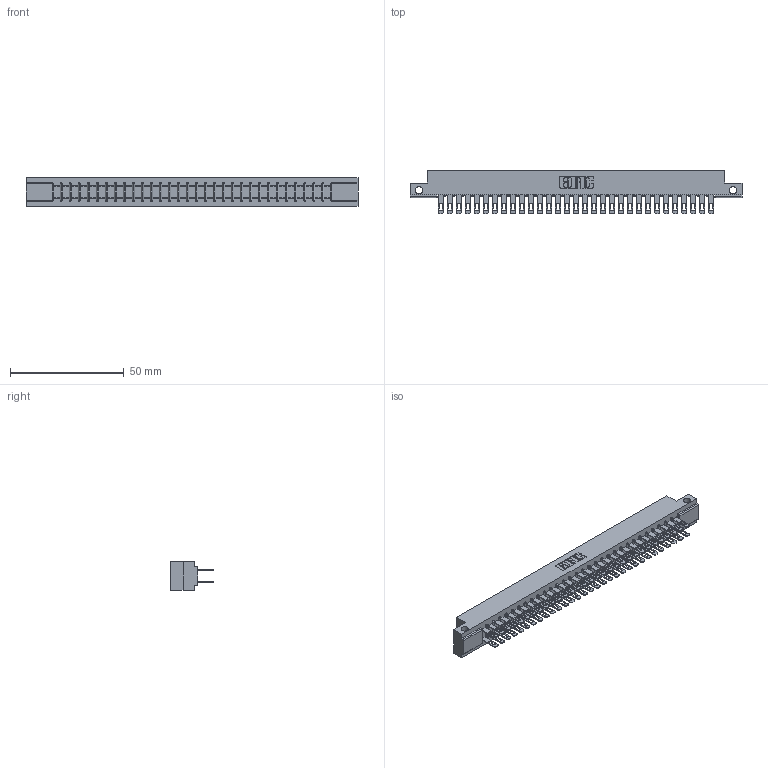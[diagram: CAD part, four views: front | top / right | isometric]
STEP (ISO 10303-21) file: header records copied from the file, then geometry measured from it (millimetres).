
FILE_DESCRIPTION (( 'STEP AP203' ), '1' );
FILE_NAME ('357-062-500-212.STEP', '2019-09-19T06:38:54', ( '' ), ( '' ), 'SwSTEP 2.0', 'SolidWorks 2016', '' );
FILE_SCHEMA (( 'CONFIG_CONTROL_DESIGN' ));
Length unit declared in the file: inch
Products named in the file (3): 357-062-500-212; 307-290-001_500; 307 Part_.128 Dia Side Mounting Holes
Assembly tree (63 placements, depth 2):
  357-062-500-212
    307 Part_.128 Dia Side Mounting Holes
    307-290-001_500  x62
Bounding box: 145.85 x 19.18 x 12.7 mm (x, y, z)
Volume: 15466.7 mm3; surface area: 19674.5 mm2
Topology: 63 solids, 63 shells, 3002 faces, 8383 edges, 5418 vertices
Faces by surface type: plane 1930, cylinder 1008, sphere 64
Entity records: 28900 total; most frequent: CARTESIAN_POINT 4727, ORIENTED_EDGE 4682, DIRECTION 4637, EDGE_CURVE 2341, LINE 1789, VECTOR 1789, VERTEX_POINT 1514, AXIS2_PLACEMENT_3D 1424
